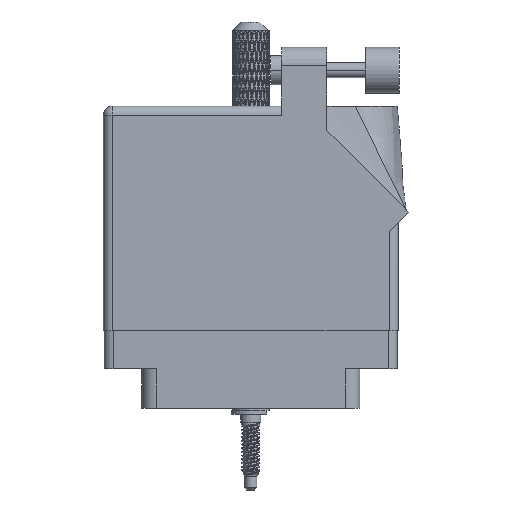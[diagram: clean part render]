
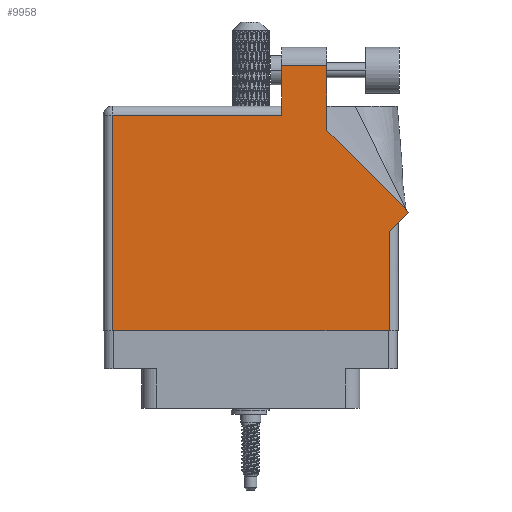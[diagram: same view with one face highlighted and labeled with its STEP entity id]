
A CAD part, front view. The second image highlights one B-rep face of the part: STEP entity #9958.
In plain terms, the highlighted face is planar.
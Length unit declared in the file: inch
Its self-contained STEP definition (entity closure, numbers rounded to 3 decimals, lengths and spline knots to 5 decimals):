
#146 = CARTESIAN_POINT ( 'NONE',  ( 1.948, 0.675, 0. ) ) ;
#1191 = DIRECTION ( 'NONE',  ( 0., 1., 0. ) ) ;
#1979 = EDGE_LOOP ( 'NONE', ( #23770, #3628, #33555, #69019, #8751, #100277, #59801, #24834, #97329 ) ) ;
#3221 = VECTOR ( 'NONE', #21551, 39.37008 ) ;
#3628 = ORIENTED_EDGE ( 'NONE', *, *, #82097, .T. ) ;
#3725 = VECTOR ( 'NONE', #55286, 39.37008 ) ;
#4828 = CARTESIAN_POINT ( 'NONE',  ( 0.062, 0., 0. ) ) ;
#5795 = CARTESIAN_POINT ( 'NONE',  ( 1.524, 1.805, 0. ) ) ;
#6594 = PLANE ( 'NONE',  #32939 ) ;
#8751 = ORIENTED_EDGE ( 'NONE', *, *, #92955, .T. ) ;
#9043 = LINE ( 'NONE', #70700, #84466 ) ;
#9630 = LINE ( 'NONE', #41270, #43696 ) ;
#9958 = ADVANCED_FACE ( 'NONE', ( #24122 ), #6594, .F. ) ;
#10540 = VERTEX_POINT ( 'NONE', #50590 ) ;
#12307 = LINE ( 'NONE', #40275, #84210 ) ;
#12383 = CARTESIAN_POINT ( 'NONE',  ( 1.524, 1.36442, 0. ) ) ;
#12595 = VERTEX_POINT ( 'NONE', #146 ) ;
#13512 = VECTOR ( 'NONE', #57620, 39.37008 ) ;
#14884 = CARTESIAN_POINT ( 'NONE',  ( 1.948, 0., 0. ) ) ;
#15076 = VECTOR ( 'NONE', #22785, 39.37008 ) ;
#15412 = EDGE_CURVE ( 'NONE', #10540, #75254, #66116, .T. ) ;
#17471 = VERTEX_POINT ( 'NONE', #4828 ) ;
#21515 = VERTEX_POINT ( 'NONE', #12383 ) ;
#21551 = DIRECTION ( 'NONE',  ( -1., 0., 0. ) ) ;
#22599 = CARTESIAN_POINT ( 'NONE',  ( 1.217, 1.468, 0. ) ) ;
#22785 = DIRECTION ( 'NONE',  ( 0., -1., 0. ) ) ;
#23770 = ORIENTED_EDGE ( 'NONE', *, *, #25372, .T. ) ;
#24122 = FACE_OUTER_BOUND ( 'NONE', #1979, .T. ) ;
#24834 = ORIENTED_EDGE ( 'NONE', *, *, #65148, .T. ) ;
#25372 = EDGE_CURVE ( 'NONE', #21515, #57692, #12307, .T. ) ;
#25740 = LINE ( 'NONE', #62689, #13512 ) ;
#29289 = VECTOR ( 'NONE', #82851, 39.37008 ) ;
#31396 = EDGE_CURVE ( 'NONE', #45433, #21515, #91339, .T. ) ;
#32939 = AXIS2_PLACEMENT_3D ( 'NONE', #45993, #37222, #99539 ) ;
#33555 = ORIENTED_EDGE ( 'NONE', *, *, #15412, .T. ) ;
#37222 = DIRECTION ( 'NONE',  ( 0., 0., -1. ) ) ;
#37551 = CARTESIAN_POINT ( 'NONE',  ( 0., 1.468, 0. ) ) ;
#38106 = CARTESIAN_POINT ( 'NONE',  ( 1.217, 1.53, 0. ) ) ;
#40275 = CARTESIAN_POINT ( 'NONE',  ( 1.524, 1.36442, 0. ) ) ;
#41270 = CARTESIAN_POINT ( 'NONE',  ( 1.948, 0.737, 0. ) ) ;
#41607 = DIRECTION ( 'NONE',  ( 0., 1., 0. ) ) ;
#43696 = VECTOR ( 'NONE', #41607, 39.37008 ) ;
#45314 = CARTESIAN_POINT ( 'NONE',  ( 2.08071, 0.80771, 0. ) ) ;
#45433 = VERTEX_POINT ( 'NONE', #45314 ) ;
#45993 = CARTESIAN_POINT ( 'NONE',  ( 0., 1.53, 0. ) ) ;
#47729 = EDGE_CURVE ( 'NONE', #74782, #12595, #9630, .T. ) ;
#48433 = DIRECTION ( 'NONE',  ( -1., 0., 0. ) ) ;
#50590 = CARTESIAN_POINT ( 'NONE',  ( 1.217, 1.805, 0. ) ) ;
#51919 = LINE ( 'NONE', #37551, #3221 ) ;
#54866 = LINE ( 'NONE', #77439, #3725 ) ;
#54932 = CARTESIAN_POINT ( 'NONE',  ( 0.062, 1.468, 0. ) ) ;
#55286 = DIRECTION ( 'NONE',  ( 0.707, 0.707, 0. ) ) ;
#57620 = DIRECTION ( 'NONE',  ( 1., 0., 0. ) ) ;
#57692 = VERTEX_POINT ( 'NONE', #5795 ) ;
#59801 = ORIENTED_EDGE ( 'NONE', *, *, #47729, .T. ) ;
#61676 = VECTOR ( 'NONE', #48433, 39.37008 ) ;
#62689 = CARTESIAN_POINT ( 'NONE',  ( 0., 0., 0. ) ) ;
#65148 = EDGE_CURVE ( 'NONE', #12595, #45433, #54866, .T. ) ;
#66116 = LINE ( 'NONE', #38106, #15076 ) ;
#68496 = CARTESIAN_POINT ( 'NONE',  ( 2.08071, 0.80771, 0. ) ) ;
#69019 = ORIENTED_EDGE ( 'NONE', *, *, #89977, .T. ) ;
#70700 = CARTESIAN_POINT ( 'NONE',  ( 0.062, 0., 0. ) ) ;
#74782 = VERTEX_POINT ( 'NONE', #14884 ) ;
#75254 = VERTEX_POINT ( 'NONE', #22599 ) ;
#77439 = CARTESIAN_POINT ( 'NONE',  ( 2.01, 0.737, 0. ) ) ;
#79452 = CARTESIAN_POINT ( 'NONE',  ( 1.217, 1.805, 0. ) ) ;
#80275 = VERTEX_POINT ( 'NONE', #54932 ) ;
#82097 = EDGE_CURVE ( 'NONE', #57692, #10540, #82421, .T. ) ;
#82421 = LINE ( 'NONE', #79452, #61676 ) ;
#82851 = DIRECTION ( 'NONE',  ( -0.707, 0.707, 0. ) ) ;
#84210 = VECTOR ( 'NONE', #1191, 39.37008 ) ;
#84466 = VECTOR ( 'NONE', #93861, 39.37008 ) ;
#89977 = EDGE_CURVE ( 'NONE', #75254, #80275, #51919, .T. ) ;
#91339 = LINE ( 'NONE', #68496, #29289 ) ;
#92955 = EDGE_CURVE ( 'NONE', #80275, #17471, #9043, .T. ) ;
#93861 = DIRECTION ( 'NONE',  ( 0., -1., 0. ) ) ;
#97329 = ORIENTED_EDGE ( 'NONE', *, *, #31396, .T. ) ;
#99539 = DIRECTION ( 'NONE',  ( -1., 0., 0. ) ) ;
#100277 = ORIENTED_EDGE ( 'NONE', *, *, #100342, .T. ) ;
#100342 = EDGE_CURVE ( 'NONE', #17471, #74782, #25740, .T. ) ;
